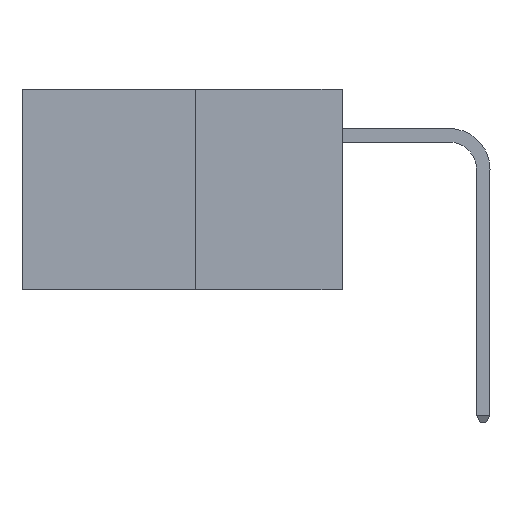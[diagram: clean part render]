
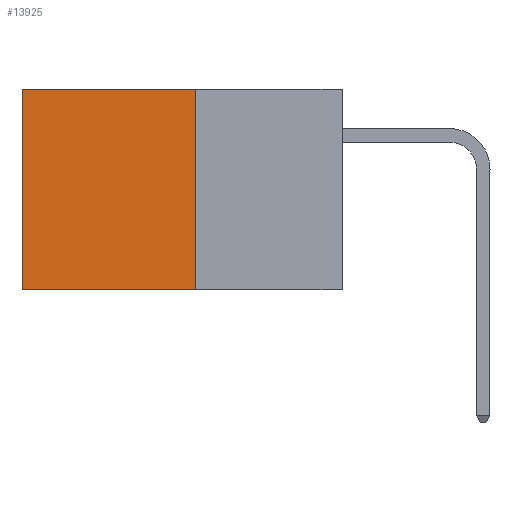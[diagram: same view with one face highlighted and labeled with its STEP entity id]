
A CAD part, left-side view. The second image highlights one B-rep face of the part: STEP entity #13925.
In plain terms, the highlighted planar face has unit normal (-1, 0, 0).
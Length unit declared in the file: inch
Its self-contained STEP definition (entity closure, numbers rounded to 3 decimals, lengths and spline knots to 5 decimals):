
#776 = CARTESIAN_POINT ( 'NONE',  ( 0.277, 0.27, 0. ) ) ;
#1970 = CARTESIAN_POINT ( 'NONE',  ( 0.277, 0.27, -0.37 ) ) ;
#2422 = CARTESIAN_POINT ( 'NONE',  ( 0.277, 0.27, -0.37 ) ) ;
#2455 = CARTESIAN_POINT ( 'NONE',  ( 0.277, 0.27, -0.37 ) ) ;
#2515 = VERTEX_POINT ( 'NONE', #12735 ) ;
#4654 = EDGE_LOOP ( 'NONE', ( #7958, #24847, #14826, #27335 ) ) ;
#4885 = DIRECTION ( 'NONE',  ( 0., 0., -1. ) ) ;
#5754 = AXIS2_PLACEMENT_3D ( 'NONE', #1970, #11563, #28424 ) ;
#6150 = VECTOR ( 'NONE', #26352, 39.37008 ) ;
#6364 = CARTESIAN_POINT ( 'NONE',  ( 0.277, 0.27, -0.37 ) ) ;
#7958 = ORIENTED_EDGE ( 'NONE', *, *, #13470, .T. ) ;
#10282 = VERTEX_POINT ( 'NONE', #12882 ) ;
#11563 = DIRECTION ( 'NONE',  ( 1., 0., 0. ) ) ;
#12019 = VECTOR ( 'NONE', #4885, 39.37008 ) ;
#12347 = CARTESIAN_POINT ( 'NONE',  ( 0.277, 0.59, -0.37 ) ) ;
#12619 = DIRECTION ( 'NONE',  ( 0., 1., 0. ) ) ;
#12735 = CARTESIAN_POINT ( 'NONE',  ( 0.277, 0.27, 0. ) ) ;
#12882 = CARTESIAN_POINT ( 'NONE',  ( 0.277, 0.59, 0. ) ) ;
#13067 = CARTESIAN_POINT ( 'NONE',  ( 0.277, 0.59, -0.37 ) ) ;
#13470 = EDGE_CURVE ( 'NONE', #10282, #13676, #17361, .T. ) ;
#13676 = VERTEX_POINT ( 'NONE', #13067 ) ;
#13925 = ADVANCED_FACE ( 'NONE', ( #16592 ), #18692, .F. ) ;
#14826 = ORIENTED_EDGE ( 'NONE', *, *, #25198, .F. ) ;
#16592 = FACE_OUTER_BOUND ( 'NONE', #4654, .T. ) ;
#17361 = LINE ( 'NONE', #12347, #23029 ) ;
#18377 = LINE ( 'NONE', #2455, #12019 ) ;
#18692 = PLANE ( 'NONE',  #5754 ) ;
#19544 = DIRECTION ( 'NONE',  ( 0., 0., -1. ) ) ;
#20773 = EDGE_CURVE ( 'NONE', #22855, #13676, #26073, .T. ) ;
#22164 = VECTOR ( 'NONE', #12619, 39.37008 ) ;
#22855 = VERTEX_POINT ( 'NONE', #6364 ) ;
#23029 = VECTOR ( 'NONE', #19544, 39.37008 ) ;
#24847 = ORIENTED_EDGE ( 'NONE', *, *, #20773, .F. ) ;
#25198 = EDGE_CURVE ( 'NONE', #2515, #22855, #18377, .T. ) ;
#26073 = LINE ( 'NONE', #2422, #6150 ) ;
#26352 = DIRECTION ( 'NONE',  ( 0., 1., 0. ) ) ;
#27335 = ORIENTED_EDGE ( 'NONE', *, *, #30263, .T. ) ;
#28424 = DIRECTION ( 'NONE',  ( 0., 0., -1. ) ) ;
#28596 = LINE ( 'NONE', #776, #22164 ) ;
#30263 = EDGE_CURVE ( 'NONE', #2515, #10282, #28596, .T. ) ;
